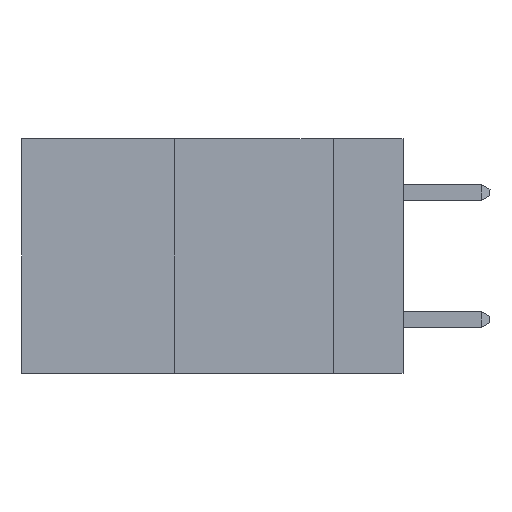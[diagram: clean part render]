
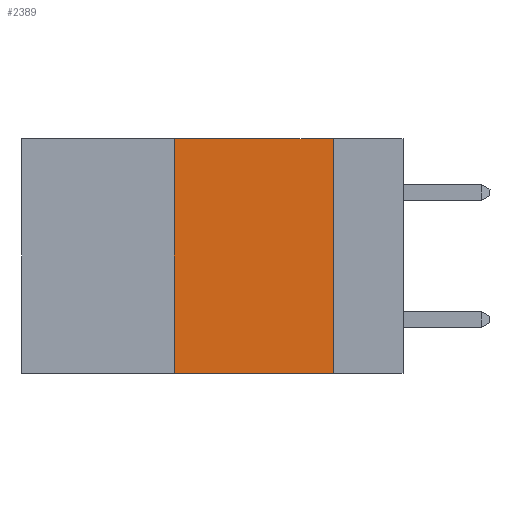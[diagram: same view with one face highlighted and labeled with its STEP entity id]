
A CAD part, left-side view. The second image highlights one B-rep face of the part: STEP entity #2389.
In plain terms, the highlighted planar face has unit normal (-1, 0, 0).
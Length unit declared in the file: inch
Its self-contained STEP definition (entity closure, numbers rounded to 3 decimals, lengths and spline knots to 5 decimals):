
#23 = VECTOR ( 'NONE', #2412, 39.37008 ) ;
#32 = CARTESIAN_POINT ( 'NONE',  ( 0., 0.11, -0.37 ) ) ;
#475 = CARTESIAN_POINT ( 'NONE',  ( 0., 0.36, 0. ) ) ;
#593 = VECTOR ( 'NONE', #9071, 39.37008 ) ;
#601 = ORIENTED_EDGE ( 'NONE', *, *, #8139, .F. ) ;
#912 = VERTEX_POINT ( 'NONE', #5406 ) ;
#1201 = AXIS2_PLACEMENT_3D ( 'NONE', #4768, #11184, #5731 ) ;
#1416 = EDGE_LOOP ( 'NONE', ( #601, #3544, #10942, #6400 ) ) ;
#1884 = PLANE ( 'NONE',  #1201 ) ;
#1973 = CARTESIAN_POINT ( 'NONE',  ( 0., 0.36, 0. ) ) ;
#2230 = LINE ( 'NONE', #10420, #11775 ) ;
#2389 = ADVANCED_FACE ( 'NONE', ( #10524 ), #1884, .F. ) ;
#2412 = DIRECTION ( 'NONE',  ( 0., 0., -1. ) ) ;
#2744 = LINE ( 'NONE', #9852, #23 ) ;
#3544 = ORIENTED_EDGE ( 'NONE', *, *, #10755, .F. ) ;
#4289 = VERTEX_POINT ( 'NONE', #5870 ) ;
#4768 = CARTESIAN_POINT ( 'NONE',  ( 0., 0.6, 0. ) ) ;
#4792 = DIRECTION ( 'NONE',  ( 0., -1., 0. ) ) ;
#4848 = VERTEX_POINT ( 'NONE', #1973 ) ;
#4887 = LINE ( 'NONE', #5750, #11589 ) ;
#4965 = VERTEX_POINT ( 'NONE', #32 ) ;
#5406 = CARTESIAN_POINT ( 'NONE',  ( 0., 0.36, -0.37 ) ) ;
#5731 = DIRECTION ( 'NONE',  ( 0., 0., -1. ) ) ;
#5750 = CARTESIAN_POINT ( 'NONE',  ( 0., 0.6, -0.37 ) ) ;
#5870 = CARTESIAN_POINT ( 'NONE',  ( 0., 0.11, 0. ) ) ;
#6297 = EDGE_CURVE ( 'NONE', #912, #4965, #4887, .T. ) ;
#6400 = ORIENTED_EDGE ( 'NONE', *, *, #6297, .T. ) ;
#6806 = DIRECTION ( 'NONE',  ( 0., -1., 0. ) ) ;
#8139 = EDGE_CURVE ( 'NONE', #4289, #4965, #2744, .T. ) ;
#8242 = LINE ( 'NONE', #475, #593 ) ;
#9071 = DIRECTION ( 'NONE',  ( 0., 0., 1. ) ) ;
#9852 = CARTESIAN_POINT ( 'NONE',  ( 0., 0.11, 0. ) ) ;
#10420 = CARTESIAN_POINT ( 'NONE',  ( 0., 0.6, 0. ) ) ;
#10524 = FACE_OUTER_BOUND ( 'NONE', #1416, .T. ) ;
#10755 = EDGE_CURVE ( 'NONE', #4848, #4289, #2230, .T. ) ;
#10942 = ORIENTED_EDGE ( 'NONE', *, *, #11892, .F. ) ;
#11184 = DIRECTION ( 'NONE',  ( 1., 0., 0. ) ) ;
#11589 = VECTOR ( 'NONE', #4792, 39.37008 ) ;
#11775 = VECTOR ( 'NONE', #6806, 39.37008 ) ;
#11892 = EDGE_CURVE ( 'NONE', #912, #4848, #8242, .T. ) ;
